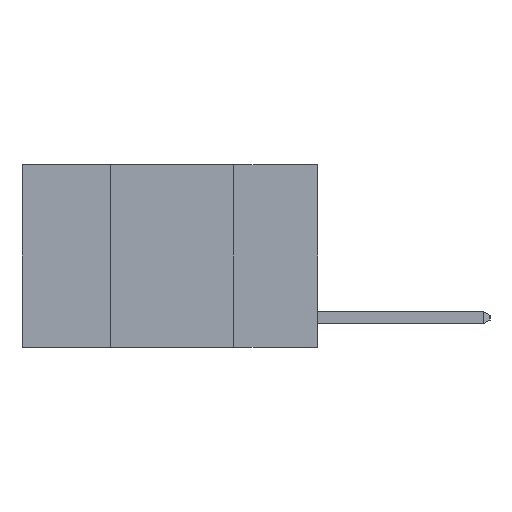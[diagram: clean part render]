
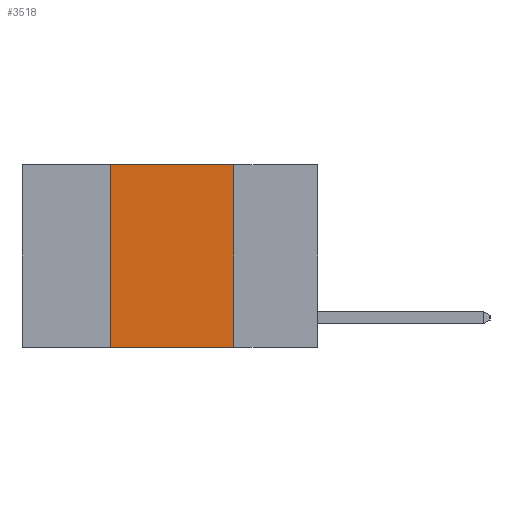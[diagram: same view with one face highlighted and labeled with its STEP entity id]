
A CAD part, left-side view. The second image highlights one B-rep face of the part: STEP entity #3518.
In plain terms, the highlighted planar face has unit normal (-1, 0, 0).
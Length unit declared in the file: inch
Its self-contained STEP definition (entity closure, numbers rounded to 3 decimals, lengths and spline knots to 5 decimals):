
#133 = ORIENTED_EDGE ( 'NONE', *, *, #4159, .F. ) ;
#177 = EDGE_LOOP ( 'NONE', ( #133, #2394, #9360, #2683 ) ) ;
#389 = CARTESIAN_POINT ( 'NONE',  ( 0., 0.17, 0. ) ) ;
#470 = VECTOR ( 'NONE', #8171, 39.37008 ) ;
#497 = VERTEX_POINT ( 'NONE', #2627 ) ;
#741 = LINE ( 'NONE', #3836, #470 ) ;
#919 = EDGE_CURVE ( 'NONE', #4445, #1327, #8244, .T. ) ;
#1327 = VERTEX_POINT ( 'NONE', #2685 ) ;
#2030 = VECTOR ( 'NONE', #6272, 39.37008 ) ;
#2390 = VECTOR ( 'NONE', #6416, 39.37008 ) ;
#2394 = ORIENTED_EDGE ( 'NONE', *, *, #7811, .F. ) ;
#2627 = CARTESIAN_POINT ( 'NONE',  ( 0., 0.42, 0. ) ) ;
#2678 = LINE ( 'NONE', #8862, #2390 ) ;
#2683 = ORIENTED_EDGE ( 'NONE', *, *, #919, .T. ) ;
#2685 = CARTESIAN_POINT ( 'NONE',  ( 0., 0.17, -0.37 ) ) ;
#3518 = ADVANCED_FACE ( 'NONE', ( #9965 ), #4502, .F. ) ;
#3615 = VECTOR ( 'NONE', #5136, 39.37008 ) ;
#3836 = CARTESIAN_POINT ( 'NONE',  ( 0., 0.6, 0. ) ) ;
#4159 = EDGE_CURVE ( 'NONE', #6277, #1327, #2678, .T. ) ;
#4407 = DIRECTION ( 'NONE',  ( 0., 0., -1. ) ) ;
#4411 = DIRECTION ( 'NONE',  ( 1., 0., 0. ) ) ;
#4445 = VERTEX_POINT ( 'NONE', #7948 ) ;
#4452 = CARTESIAN_POINT ( 'NONE',  ( 0., 0.6, 0. ) ) ;
#4502 = PLANE ( 'NONE',  #10152 ) ;
#5136 = DIRECTION ( 'NONE',  ( 0., -1., 0. ) ) ;
#5423 = CARTESIAN_POINT ( 'NONE',  ( 0., 0.42, 0. ) ) ;
#5532 = CARTESIAN_POINT ( 'NONE',  ( 0., 0.6, -0.37 ) ) ;
#6272 = DIRECTION ( 'NONE',  ( 0., 0., 1. ) ) ;
#6277 = VERTEX_POINT ( 'NONE', #389 ) ;
#6416 = DIRECTION ( 'NONE',  ( 0., 0., -1. ) ) ;
#7811 = EDGE_CURVE ( 'NONE', #497, #6277, #741, .T. ) ;
#7948 = CARTESIAN_POINT ( 'NONE',  ( 0., 0.42, -0.37 ) ) ;
#8171 = DIRECTION ( 'NONE',  ( 0., -1., 0. ) ) ;
#8244 = LINE ( 'NONE', #5532, #3615 ) ;
#8767 = LINE ( 'NONE', #5423, #2030 ) ;
#8862 = CARTESIAN_POINT ( 'NONE',  ( 0., 0.17, 0. ) ) ;
#9264 = EDGE_CURVE ( 'NONE', #4445, #497, #8767, .T. ) ;
#9360 = ORIENTED_EDGE ( 'NONE', *, *, #9264, .F. ) ;
#9965 = FACE_OUTER_BOUND ( 'NONE', #177, .T. ) ;
#10152 = AXIS2_PLACEMENT_3D ( 'NONE', #4452, #4411, #4407 ) ;
